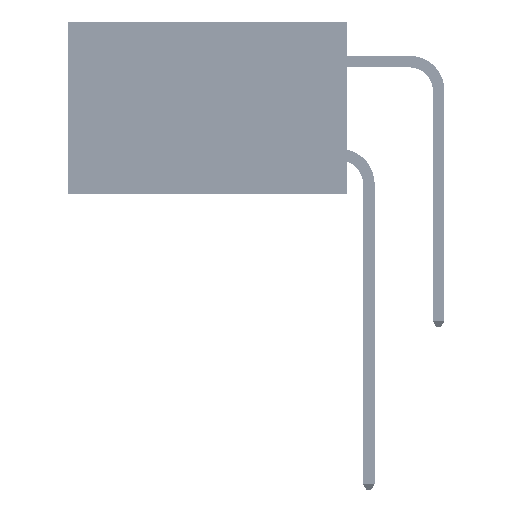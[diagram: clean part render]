
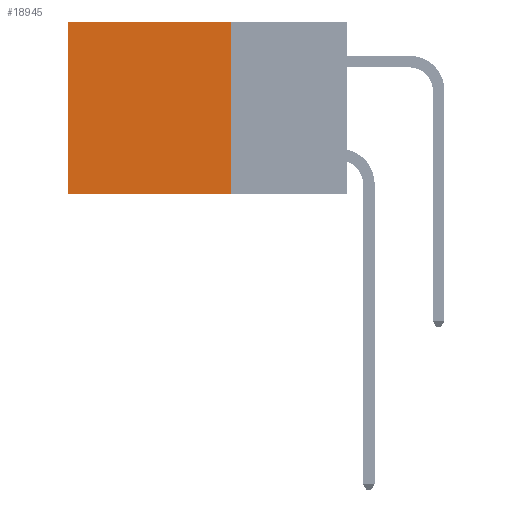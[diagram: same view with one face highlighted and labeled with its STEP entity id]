
A CAD part, left-side view. The second image highlights one B-rep face of the part: STEP entity #18945.
In plain terms, the highlighted planar face has unit normal (-1, 0, 0).
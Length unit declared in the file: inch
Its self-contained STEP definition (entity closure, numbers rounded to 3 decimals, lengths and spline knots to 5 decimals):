
#4808 = VECTOR ( 'NONE', #10576, 39.37008 ) ;
#5244 = FACE_OUTER_BOUND ( 'NONE', #31036, .T. ) ;
#6557 = VERTEX_POINT ( 'NONE', #19107 ) ;
#8519 = CARTESIAN_POINT ( 'NONE',  ( 0.2875, 0.6, 0. ) ) ;
#8857 = PLANE ( 'NONE',  #14529 ) ;
#9260 = EDGE_CURVE ( 'NONE', #37364, #9917, #35035, .T. ) ;
#9917 = VERTEX_POINT ( 'NONE', #47287 ) ;
#10576 = DIRECTION ( 'NONE',  ( 0., 1., 0. ) ) ;
#11156 = CARTESIAN_POINT ( 'NONE',  ( 0.2875, 0.6, 0. ) ) ;
#12964 = LINE ( 'NONE', #43806, #31864 ) ;
#14529 = AXIS2_PLACEMENT_3D ( 'NONE', #16821, #43104, #20610 ) ;
#15025 = VECTOR ( 'NONE', #41421, 39.37008 ) ;
#16821 = CARTESIAN_POINT ( 'NONE',  ( 0.2875, 0.25, 0. ) ) ;
#18394 = EDGE_CURVE ( 'NONE', #21020, #37364, #12964, .T. ) ;
#18945 = ADVANCED_FACE ( 'NONE', ( #5244 ), #8857, .F. ) ;
#19107 = CARTESIAN_POINT ( 'NONE',  ( 0.2875, 0.25, -0.37 ) ) ;
#20610 = DIRECTION ( 'NONE',  ( 0., 0., -1. ) ) ;
#21020 = VERTEX_POINT ( 'NONE', #45239 ) ;
#21798 = CARTESIAN_POINT ( 'NONE',  ( 0.2875, 0.25, -0.37 ) ) ;
#23552 = DIRECTION ( 'NONE',  ( 0., 0., -1. ) ) ;
#23720 = CARTESIAN_POINT ( 'NONE',  ( 0.2875, 0.25, 0. ) ) ;
#25897 = ORIENTED_EDGE ( 'NONE', *, *, #18394, .T. ) ;
#26164 = ORIENTED_EDGE ( 'NONE', *, *, #45817, .F. ) ;
#27191 = EDGE_CURVE ( 'NONE', #6557, #9917, #34960, .T. ) ;
#30354 = LINE ( 'NONE', #23720, #40310 ) ;
#31036 = EDGE_LOOP ( 'NONE', ( #41349, #37682, #26164, #25897 ) ) ;
#31864 = VECTOR ( 'NONE', #40034, 39.37008 ) ;
#34960 = LINE ( 'NONE', #21798, #4808 ) ;
#35035 = LINE ( 'NONE', #11156, #15025 ) ;
#37364 = VERTEX_POINT ( 'NONE', #8519 ) ;
#37682 = ORIENTED_EDGE ( 'NONE', *, *, #27191, .F. ) ;
#40034 = DIRECTION ( 'NONE',  ( 0., 1., 0. ) ) ;
#40310 = VECTOR ( 'NONE', #23552, 39.37008 ) ;
#41349 = ORIENTED_EDGE ( 'NONE', *, *, #9260, .T. ) ;
#41421 = DIRECTION ( 'NONE',  ( 0., 0., -1. ) ) ;
#43104 = DIRECTION ( 'NONE',  ( 1., 0., 0. ) ) ;
#43806 = CARTESIAN_POINT ( 'NONE',  ( 0.2875, 0.25, 0. ) ) ;
#45239 = CARTESIAN_POINT ( 'NONE',  ( 0.2875, 0.25, 0. ) ) ;
#45817 = EDGE_CURVE ( 'NONE', #21020, #6557, #30354, .T. ) ;
#47287 = CARTESIAN_POINT ( 'NONE',  ( 0.2875, 0.6, -0.37 ) ) ;
